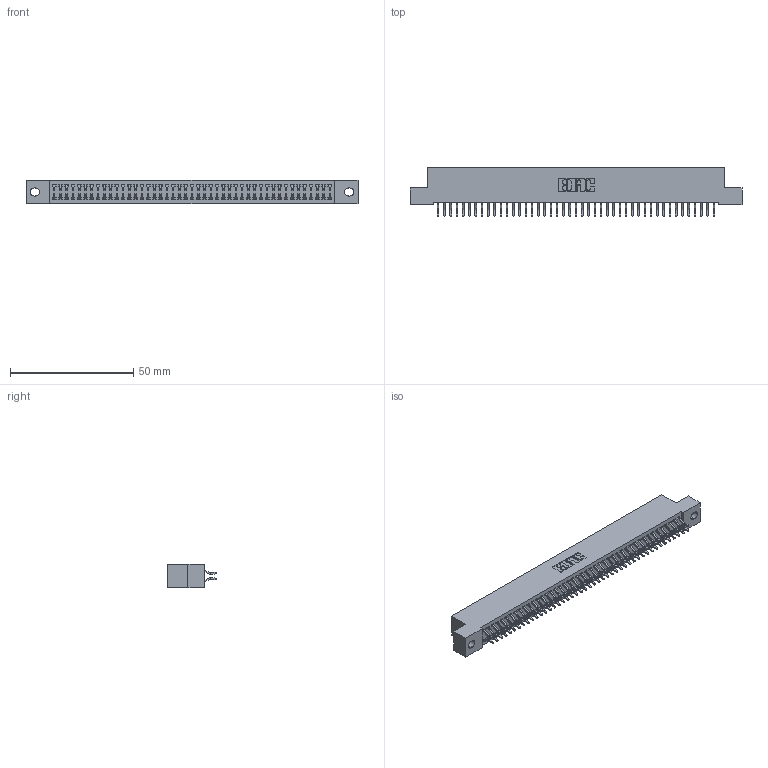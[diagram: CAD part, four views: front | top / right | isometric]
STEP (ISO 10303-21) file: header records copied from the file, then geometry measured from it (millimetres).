
FILE_DESCRIPTION (( 'STEP AP203' ), '1' );
FILE_NAME ('392-090-556-202.STEP', '2018-08-18T07:19:42', ( '' ), ( '' ), 'SwSTEP 2.0', 'SolidWorks 2016', '' );
FILE_SCHEMA (( 'CONFIG_CONTROL_DESIGN' ));
Length unit declared in the file: inch
Products named in the file (3): 345-292-001_556 Tail; 392-090-556-202; 342 Part_.128 Slot
Assembly tree (91 placements, depth 2):
  392-090-556-202
    342 Part_.128 Slot
    345-292-001_556 Tail  x90
Bounding box: 134.62 x 19.58 x 9.4 mm (x, y, z)
Volume: 12055.4 mm3; surface area: 19369.2 mm2
Topology: 91 solids, 91 shells, 5334 faces, 15881 edges, 10466 vertices
Faces by surface type: plane 3670, cylinder 1664
Entity records: 28785 total; most frequent: CARTESIAN_POINT 4782, ORIENTED_EDGE 4706, DIRECTION 4069, EDGE_CURVE 2353, LINE 2217, VECTOR 2217, VERTEX_POINT 1566, AXIS2_PLACEMENT_3D 926
